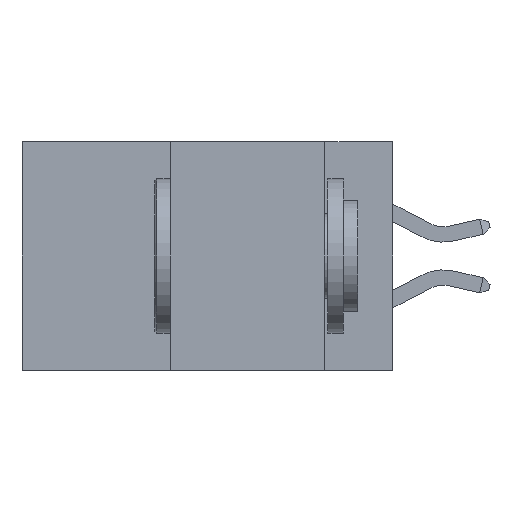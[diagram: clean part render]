
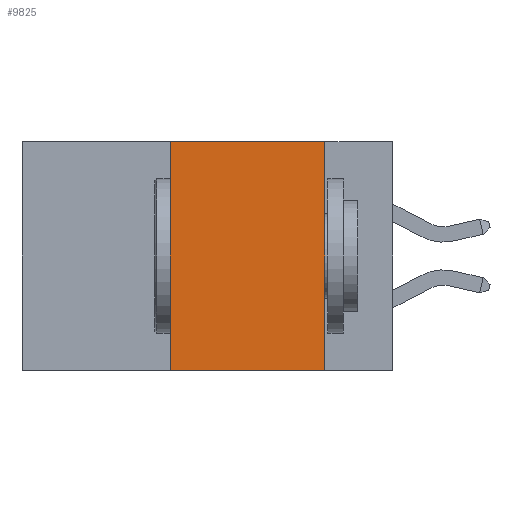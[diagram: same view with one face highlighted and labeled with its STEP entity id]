
A CAD part, left-side view. The second image highlights one B-rep face of the part: STEP entity #9825.
In plain terms, the highlighted planar face has unit normal (-1, 0, 0).
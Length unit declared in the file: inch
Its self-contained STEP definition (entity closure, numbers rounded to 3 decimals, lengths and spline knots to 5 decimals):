
#243 = CARTESIAN_POINT ( 'NONE',  ( 0., 0.36, 0. ) ) ;
#371 = CARTESIAN_POINT ( 'NONE',  ( 0., 0.36, 0. ) ) ;
#524 = EDGE_LOOP ( 'NONE', ( #16251, #6206, #13360, #18241 ) ) ;
#794 = DIRECTION ( 'NONE',  ( 1., 0., 0. ) ) ;
#1058 = VECTOR ( 'NONE', #7175, 39.37008 ) ;
#2210 = DIRECTION ( 'NONE',  ( 0., 0., -1. ) ) ;
#3151 = LINE ( 'NONE', #5882, #10306 ) ;
#3310 = FACE_OUTER_BOUND ( 'NONE', #524, .T. ) ;
#4843 = VECTOR ( 'NONE', #6119, 39.37008 ) ;
#5616 = CARTESIAN_POINT ( 'NONE',  ( 0., 0.6, -0.37 ) ) ;
#5882 = CARTESIAN_POINT ( 'NONE',  ( 0., 0.6, 0. ) ) ;
#6119 = DIRECTION ( 'NONE',  ( 0., 0., 1. ) ) ;
#6206 = ORIENTED_EDGE ( 'NONE', *, *, #12969, .F. ) ;
#6558 = VERTEX_POINT ( 'NONE', #8658 ) ;
#6638 = CARTESIAN_POINT ( 'NONE',  ( 0., 0.11, 0. ) ) ;
#6686 = VERTEX_POINT ( 'NONE', #371 ) ;
#7175 = DIRECTION ( 'NONE',  ( 0., -1., 0. ) ) ;
#7637 = EDGE_CURVE ( 'NONE', #16941, #6686, #16139, .T. ) ;
#7682 = CARTESIAN_POINT ( 'NONE',  ( 0., 0.11, 0. ) ) ;
#7727 = LINE ( 'NONE', #6638, #14325 ) ;
#8526 = EDGE_CURVE ( 'NONE', #16082, #6558, #7727, .T. ) ;
#8658 = CARTESIAN_POINT ( 'NONE',  ( 0., 0.11, -0.37 ) ) ;
#8959 = DIRECTION ( 'NONE',  ( 0., -1., 0. ) ) ;
#9825 = ADVANCED_FACE ( 'NONE', ( #3310 ), #12168, .F. ) ;
#10306 = VECTOR ( 'NONE', #8959, 39.37008 ) ;
#10808 = EDGE_CURVE ( 'NONE', #16941, #6558, #16364, .T. ) ;
#12168 = PLANE ( 'NONE',  #14047 ) ;
#12969 = EDGE_CURVE ( 'NONE', #6686, #16082, #3151, .T. ) ;
#13360 = ORIENTED_EDGE ( 'NONE', *, *, #7637, .F. ) ;
#14047 = AXIS2_PLACEMENT_3D ( 'NONE', #15112, #794, #16363 ) ;
#14325 = VECTOR ( 'NONE', #2210, 39.37008 ) ;
#15112 = CARTESIAN_POINT ( 'NONE',  ( 0., 0.6, 0. ) ) ;
#15478 = CARTESIAN_POINT ( 'NONE',  ( 0., 0.36, -0.37 ) ) ;
#16082 = VERTEX_POINT ( 'NONE', #7682 ) ;
#16139 = LINE ( 'NONE', #243, #4843 ) ;
#16251 = ORIENTED_EDGE ( 'NONE', *, *, #8526, .F. ) ;
#16363 = DIRECTION ( 'NONE',  ( 0., 0., -1. ) ) ;
#16364 = LINE ( 'NONE', #5616, #1058 ) ;
#16941 = VERTEX_POINT ( 'NONE', #15478 ) ;
#18241 = ORIENTED_EDGE ( 'NONE', *, *, #10808, .T. ) ;
